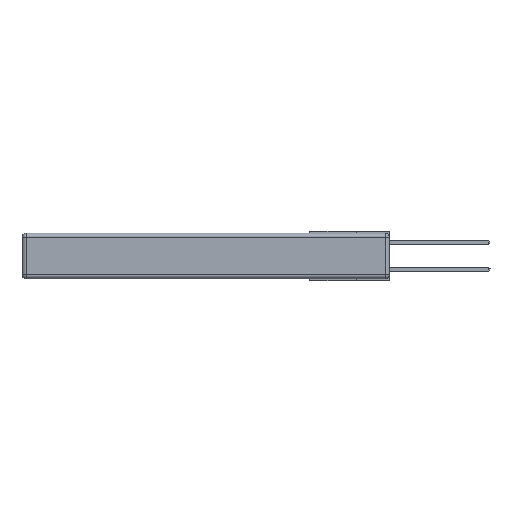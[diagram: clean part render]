
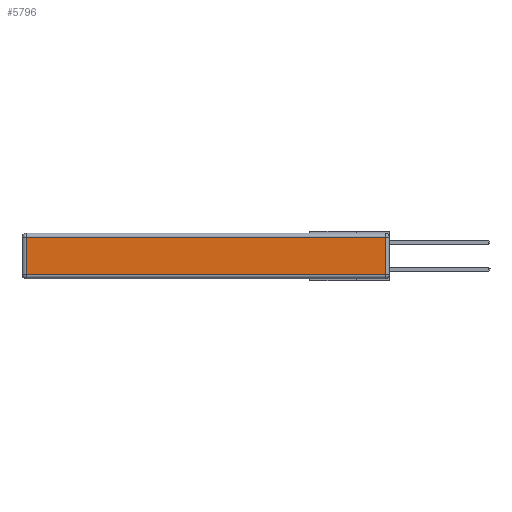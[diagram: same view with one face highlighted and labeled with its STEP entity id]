
A CAD part, left-side view. The second image highlights one B-rep face of the part: STEP entity #5796.
In plain terms, the highlighted planar face has unit normal (-1, 0, 0).
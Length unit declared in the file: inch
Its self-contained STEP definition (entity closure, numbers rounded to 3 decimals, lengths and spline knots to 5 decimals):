
#79 = EDGE_LOOP ( 'NONE', ( #12298, #5873, #7999, #671 ) ) ;
#657 = CARTESIAN_POINT ( 'NONE',  ( 0., 2.72, -0.343 ) ) ;
#671 = ORIENTED_EDGE ( 'NONE', *, *, #4712, .T. ) ;
#1355 = LINE ( 'NONE', #8966, #8308 ) ;
#1411 = CARTESIAN_POINT ( 'NONE',  ( 0., 2.72, -0.03 ) ) ;
#1962 = DIRECTION ( 'NONE',  ( 0., 1., 0. ) ) ;
#2060 = AXIS2_PLACEMENT_3D ( 'NONE', #14746, #2912, #7600 ) ;
#2330 = VERTEX_POINT ( 'NONE', #12265 ) ;
#2359 = CARTESIAN_POINT ( 'NONE',  ( 0., 0.03, -0.03 ) ) ;
#2613 = CARTESIAN_POINT ( 'NONE',  ( 0., 0., -0.313 ) ) ;
#2912 = DIRECTION ( 'NONE',  ( -1., 0., 0. ) ) ;
#3020 = DIRECTION ( 'NONE',  ( 0., 0., -1. ) ) ;
#3399 = VECTOR ( 'NONE', #3020, 39.37008 ) ;
#4712 = EDGE_CURVE ( 'NONE', #4779, #2330, #9619, .T. ) ;
#4779 = VERTEX_POINT ( 'NONE', #1411 ) ;
#4929 = EDGE_CURVE ( 'NONE', #12879, #4779, #1355, .T. ) ;
#5796 = ADVANCED_FACE ( 'NONE', ( #7750 ), #12428, .T. ) ;
#5873 = ORIENTED_EDGE ( 'NONE', *, *, #12772, .T. ) ;
#6022 = DIRECTION ( 'NONE',  ( 0., -1., 0. ) ) ;
#7600 = DIRECTION ( 'NONE',  ( 0., 0., 1. ) ) ;
#7750 = FACE_OUTER_BOUND ( 'NONE', #79, .T. ) ;
#7991 = LINE ( 'NONE', #10319, #14381 ) ;
#7999 = ORIENTED_EDGE ( 'NONE', *, *, #4929, .T. ) ;
#8308 = VECTOR ( 'NONE', #1962, 39.37008 ) ;
#8461 = EDGE_CURVE ( 'NONE', #2330, #8710, #14806, .T. ) ;
#8710 = VERTEX_POINT ( 'NONE', #14844 ) ;
#8966 = CARTESIAN_POINT ( 'NONE',  ( 0., 2.75, -0.03 ) ) ;
#9619 = LINE ( 'NONE', #657, #3399 ) ;
#10319 = CARTESIAN_POINT ( 'NONE',  ( 0., 0.03, -0.343 ) ) ;
#12265 = CARTESIAN_POINT ( 'NONE',  ( 0., 2.72, -0.313 ) ) ;
#12298 = ORIENTED_EDGE ( 'NONE', *, *, #8461, .T. ) ;
#12428 = PLANE ( 'NONE',  #2060 ) ;
#12772 = EDGE_CURVE ( 'NONE', #8710, #12879, #7991, .T. ) ;
#12879 = VERTEX_POINT ( 'NONE', #2359 ) ;
#12996 = VECTOR ( 'NONE', #6022, 39.37008 ) ;
#14381 = VECTOR ( 'NONE', #14913, 39.37008 ) ;
#14746 = CARTESIAN_POINT ( 'NONE',  ( 0., 0., -0.343 ) ) ;
#14806 = LINE ( 'NONE', #2613, #12996 ) ;
#14844 = CARTESIAN_POINT ( 'NONE',  ( 0., 0.03, -0.313 ) ) ;
#14913 = DIRECTION ( 'NONE',  ( 0., 0., 1. ) ) ;
